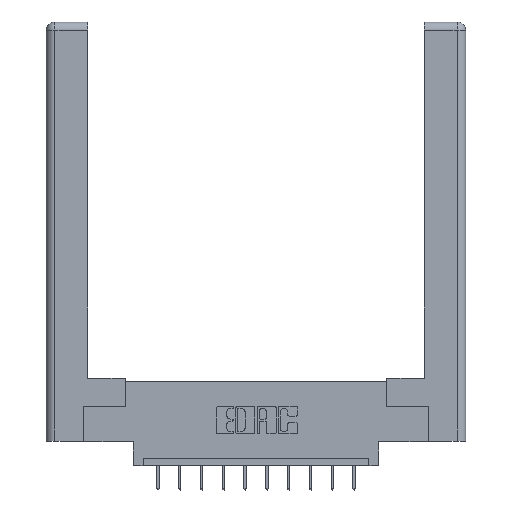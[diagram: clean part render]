
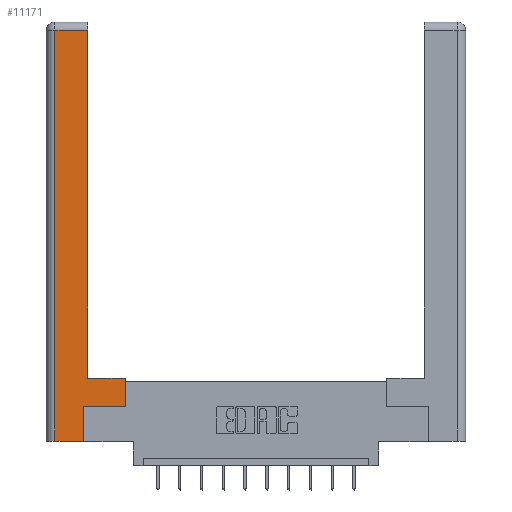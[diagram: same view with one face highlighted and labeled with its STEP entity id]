
A CAD part, top view. The second image highlights one B-rep face of the part: STEP entity #11171.
In plain terms, the highlighted planar face has unit normal (0, 0, 1).
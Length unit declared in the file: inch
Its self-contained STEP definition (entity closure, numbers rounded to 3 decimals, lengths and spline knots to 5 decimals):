
#492 = CARTESIAN_POINT ( 'NONE',  ( 0.565, 0.245, 0. ) ) ;
#504 = VERTEX_POINT ( 'NONE', #10730 ) ;
#590 = VECTOR ( 'NONE', #1606, 39.37008 ) ;
#667 = VECTOR ( 'NONE', #5418, 39.37008 ) ;
#764 = EDGE_CURVE ( 'NONE', #6675, #3758, #4718, .T. ) ;
#853 = LINE ( 'NONE', #492, #12350 ) ;
#860 = CARTESIAN_POINT ( 'NONE',  ( 0.565, 0.45, 0. ) ) ;
#955 = DIRECTION ( 'NONE',  ( -1., 0., 0. ) ) ;
#1005 = LINE ( 'NONE', #12069, #667 ) ;
#1282 = EDGE_CURVE ( 'NONE', #13999, #6675, #1005, .T. ) ;
#1304 = CARTESIAN_POINT ( 'NONE',  ( 0.0615, 2.94, 0. ) ) ;
#1338 = DIRECTION ( 'NONE',  ( 0., 1., 0. ) ) ;
#1437 = EDGE_LOOP ( 'NONE', ( #5729, #10527, #8380, #8950, #13897, #13501, #4977, #4636 ) ) ;
#1606 = DIRECTION ( 'NONE',  ( 0., 1., 0. ) ) ;
#1608 = FACE_OUTER_BOUND ( 'NONE', #1437, .T. ) ;
#1684 = LINE ( 'NONE', #4250, #5527 ) ;
#1735 = VECTOR ( 'NONE', #11881, 39.37008 ) ;
#2155 = EDGE_CURVE ( 'NONE', #504, #13999, #1684, .T. ) ;
#2600 = AXIS2_PLACEMENT_3D ( 'NONE', #3295, #11060, #11254 ) ;
#3295 = CARTESIAN_POINT ( 'NONE',  ( 0., 0., 0. ) ) ;
#3758 = VERTEX_POINT ( 'NONE', #11604 ) ;
#3904 = VECTOR ( 'NONE', #1338, 39.37008 ) ;
#4004 = EDGE_CURVE ( 'NONE', #11918, #504, #13648, .T. ) ;
#4019 = CARTESIAN_POINT ( 'NONE',  ( 0.295, 0.45, 0. ) ) ;
#4250 = CARTESIAN_POINT ( 'NONE',  ( 0.0615, 2.94, 0. ) ) ;
#4252 = LINE ( 'NONE', #13529, #10497 ) ;
#4636 = ORIENTED_EDGE ( 'NONE', *, *, #6759, .T. ) ;
#4693 = CARTESIAN_POINT ( 'NONE',  ( 0.265, 0., 0. ) ) ;
#4718 = LINE ( 'NONE', #4693, #1735 ) ;
#4977 = ORIENTED_EDGE ( 'NONE', *, *, #10029, .T. ) ;
#5418 = DIRECTION ( 'NONE',  ( 0., -1., 0. ) ) ;
#5527 = VECTOR ( 'NONE', #14084, 39.37008 ) ;
#5729 = ORIENTED_EDGE ( 'NONE', *, *, #4004, .T. ) ;
#6219 = CARTESIAN_POINT ( 'NONE',  ( 0.0615, 0., 0. ) ) ;
#6603 = VERTEX_POINT ( 'NONE', #13090 ) ;
#6675 = VERTEX_POINT ( 'NONE', #6219 ) ;
#6759 = EDGE_CURVE ( 'NONE', #8862, #11918, #10248, .T. ) ;
#6885 = LINE ( 'NONE', #13579, #3904 ) ;
#7085 = DIRECTION ( 'NONE',  ( 1., 0., 0. ) ) ;
#7320 = VECTOR ( 'NONE', #955, 39.37008 ) ;
#8380 = ORIENTED_EDGE ( 'NONE', *, *, #1282, .T. ) ;
#8862 = VERTEX_POINT ( 'NONE', #860 ) ;
#8950 = ORIENTED_EDGE ( 'NONE', *, *, #764, .T. ) ;
#10022 = EDGE_CURVE ( 'NONE', #3758, #10111, #6885, .T. ) ;
#10029 = EDGE_CURVE ( 'NONE', #6603, #8862, #4252, .T. ) ;
#10111 = VERTEX_POINT ( 'NONE', #11354 ) ;
#10248 = LINE ( 'NONE', #13152, #7320 ) ;
#10497 = VECTOR ( 'NONE', #11301, 39.37008 ) ;
#10527 = ORIENTED_EDGE ( 'NONE', *, *, #2155, .T. ) ;
#10730 = CARTESIAN_POINT ( 'NONE',  ( 0.295, 2.94, 0. ) ) ;
#11060 = DIRECTION ( 'NONE',  ( 0., 0., -1. ) ) ;
#11171 = ADVANCED_FACE ( 'NONE', ( #1608 ), #13476, .F. ) ;
#11254 = DIRECTION ( 'NONE',  ( -1., 0., 0. ) ) ;
#11301 = DIRECTION ( 'NONE',  ( 0., 1., 0. ) ) ;
#11354 = CARTESIAN_POINT ( 'NONE',  ( 0.265, 0.245, 0. ) ) ;
#11604 = CARTESIAN_POINT ( 'NONE',  ( 0.265, 0., 0. ) ) ;
#11881 = DIRECTION ( 'NONE',  ( 1., 0., 0. ) ) ;
#11918 = VERTEX_POINT ( 'NONE', #4019 ) ;
#12069 = CARTESIAN_POINT ( 'NONE',  ( 0.0615, 0., 0. ) ) ;
#12301 = EDGE_CURVE ( 'NONE', #10111, #6603, #853, .T. ) ;
#12350 = VECTOR ( 'NONE', #7085, 39.37008 ) ;
#13090 = CARTESIAN_POINT ( 'NONE',  ( 0.565, 0.245, 0. ) ) ;
#13152 = CARTESIAN_POINT ( 'NONE',  ( 0.295, 0.45, 0. ) ) ;
#13476 = PLANE ( 'NONE',  #2600 ) ;
#13501 = ORIENTED_EDGE ( 'NONE', *, *, #12301, .T. ) ;
#13529 = CARTESIAN_POINT ( 'NONE',  ( 0.565, 0.45, 0. ) ) ;
#13579 = CARTESIAN_POINT ( 'NONE',  ( 0.265, 0.245, 0. ) ) ;
#13643 = CARTESIAN_POINT ( 'NONE',  ( 0.295, 3., 0. ) ) ;
#13648 = LINE ( 'NONE', #13643, #590 ) ;
#13897 = ORIENTED_EDGE ( 'NONE', *, *, #10022, .T. ) ;
#13999 = VERTEX_POINT ( 'NONE', #1304 ) ;
#14084 = DIRECTION ( 'NONE',  ( -1., 0., 0. ) ) ;
